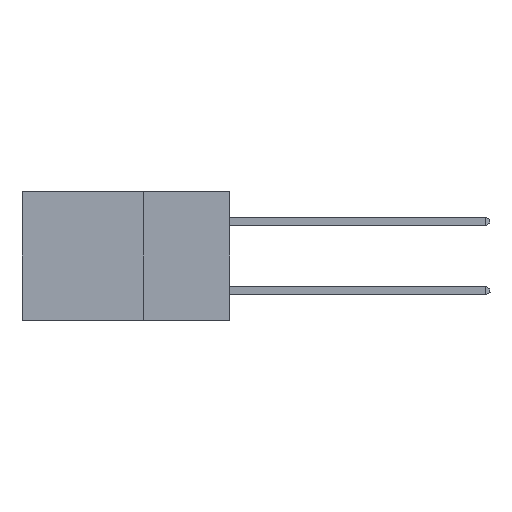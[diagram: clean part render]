
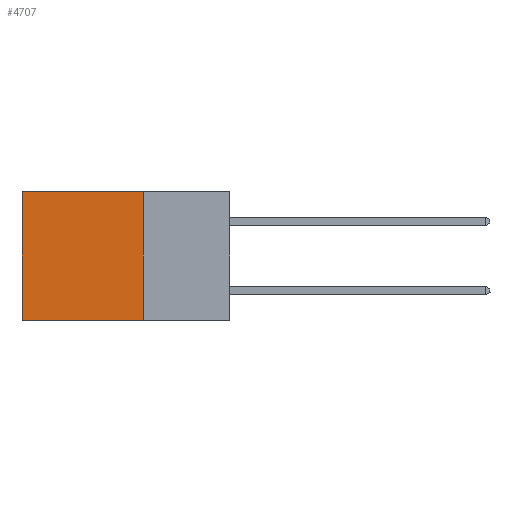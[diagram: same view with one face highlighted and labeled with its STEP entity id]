
A CAD part, left-side view. The second image highlights one B-rep face of the part: STEP entity #4707.
In plain terms, the highlighted planar face has unit normal (-1, 0, 0).
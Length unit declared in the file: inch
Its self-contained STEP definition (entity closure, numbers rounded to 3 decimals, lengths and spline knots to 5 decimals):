
#219 = ORIENTED_EDGE ( 'NONE', *, *, #20169, .T. ) ;
#1462 = DIRECTION ( 'NONE',  ( 0., 1., 0. ) ) ;
#1522 = ORIENTED_EDGE ( 'NONE', *, *, #4221, .F. ) ;
#1816 = DIRECTION ( 'NONE',  ( 1., 0., 0. ) ) ;
#2626 = DIRECTION ( 'NONE',  ( 0., 1., 0. ) ) ;
#2671 = VERTEX_POINT ( 'NONE', #12802 ) ;
#4221 = EDGE_CURVE ( 'NONE', #27542, #2671, #11895, .T. ) ;
#4707 = ADVANCED_FACE ( 'NONE', ( #10367 ), #6663, .F. ) ;
#6432 = CARTESIAN_POINT ( 'NONE',  ( 0.298, 0.25, 0. ) ) ;
#6663 = PLANE ( 'NONE',  #8906 ) ;
#6736 = VERTEX_POINT ( 'NONE', #21358 ) ;
#6936 = LINE ( 'NONE', #7003, #12604 ) ;
#6989 = DIRECTION ( 'NONE',  ( 0., 0., -1. ) ) ;
#7003 = CARTESIAN_POINT ( 'NONE',  ( 0.298, 0.6, 0. ) ) ;
#7401 = ORIENTED_EDGE ( 'NONE', *, *, #26853, .F. ) ;
#7474 = ORIENTED_EDGE ( 'NONE', *, *, #9898, .T. ) ;
#8906 = AXIS2_PLACEMENT_3D ( 'NONE', #16378, #1816, #18762 ) ;
#9898 = EDGE_CURVE ( 'NONE', #6736, #13355, #18110, .T. ) ;
#10367 = FACE_OUTER_BOUND ( 'NONE', #17235, .T. ) ;
#11895 = LINE ( 'NONE', #26564, #12650 ) ;
#12604 = VECTOR ( 'NONE', #23727, 39.37008 ) ;
#12650 = VECTOR ( 'NONE', #2626, 39.37008 ) ;
#12802 = CARTESIAN_POINT ( 'NONE',  ( 0.298, 0.6, -0.37 ) ) ;
#13355 = VERTEX_POINT ( 'NONE', #29756 ) ;
#13767 = VECTOR ( 'NONE', #6989, 39.37008 ) ;
#14519 = LINE ( 'NONE', #23713, #13767 ) ;
#16378 = CARTESIAN_POINT ( 'NONE',  ( 0.298, 0.25, 0. ) ) ;
#17235 = EDGE_LOOP ( 'NONE', ( #219, #1522, #7401, #7474 ) ) ;
#17360 = VECTOR ( 'NONE', #1462, 39.37008 ) ;
#18110 = LINE ( 'NONE', #6432, #17360 ) ;
#18762 = DIRECTION ( 'NONE',  ( 0., 0., -1. ) ) ;
#20169 = EDGE_CURVE ( 'NONE', #13355, #2671, #6936, .T. ) ;
#21358 = CARTESIAN_POINT ( 'NONE',  ( 0.298, 0.25, 0. ) ) ;
#23713 = CARTESIAN_POINT ( 'NONE',  ( 0.298, 0.25, 0. ) ) ;
#23727 = DIRECTION ( 'NONE',  ( 0., 0., -1. ) ) ;
#25887 = CARTESIAN_POINT ( 'NONE',  ( 0.298, 0.25, -0.37 ) ) ;
#26564 = CARTESIAN_POINT ( 'NONE',  ( 0.298, 0.25, -0.37 ) ) ;
#26853 = EDGE_CURVE ( 'NONE', #6736, #27542, #14519, .T. ) ;
#27542 = VERTEX_POINT ( 'NONE', #25887 ) ;
#29756 = CARTESIAN_POINT ( 'NONE',  ( 0.298, 0.6, 0. ) ) ;
